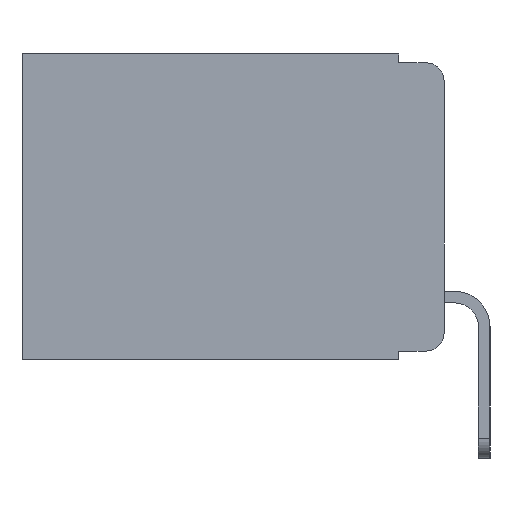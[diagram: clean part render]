
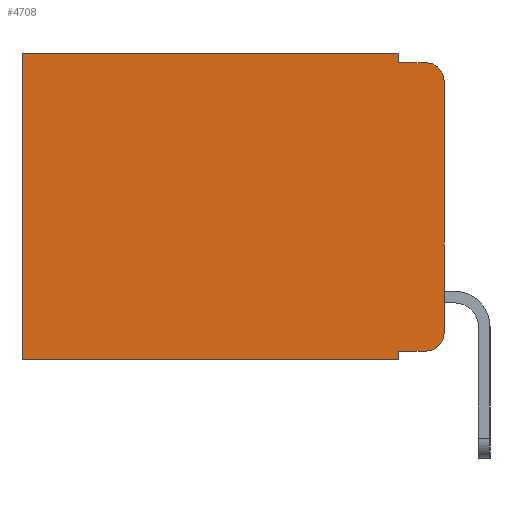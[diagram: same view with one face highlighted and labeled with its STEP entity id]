
A CAD part, left-side view. The second image highlights one B-rep face of the part: STEP entity #4708.
In plain terms, the highlighted planar face has unit normal (-1, 0, 0).
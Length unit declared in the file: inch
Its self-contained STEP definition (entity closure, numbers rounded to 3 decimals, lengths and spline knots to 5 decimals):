
#97 = VERTEX_POINT ( 'NONE', #3400 ) ;
#129 = EDGE_CURVE ( 'NONE', #6507, #97, #11441, .T. ) ;
#184 = VECTOR ( 'NONE', #4500, 39.37008 ) ;
#549 = CARTESIAN_POINT ( 'NONE',  ( 0.298, 0.02, -0.03 ) ) ;
#659 = CARTESIAN_POINT ( 'NONE',  ( 0.298, 0.473, 0. ) ) ;
#686 = LINE ( 'NONE', #10737, #2802 ) ;
#793 = CARTESIAN_POINT ( 'NONE',  ( 0.298, 0.051, -0.333 ) ) ;
#850 = EDGE_CURVE ( 'NONE', #11852, #7613, #6948, .T. ) ;
#1133 = VERTEX_POINT ( 'NONE', #4313 ) ;
#1207 = CARTESIAN_POINT ( 'NONE',  ( 0.298, 0.051, -0.01 ) ) ;
#1208 = VECTOR ( 'NONE', #5423, 39.37008 ) ;
#1633 = ORIENTED_EDGE ( 'NONE', *, *, #5305, .F. ) ;
#1753 = EDGE_CURVE ( 'NONE', #10058, #8512, #686, .T. ) ;
#1862 = LINE ( 'NONE', #9251, #4574 ) ;
#1999 = DIRECTION ( 'NONE',  ( 0., 0., -1. ) ) ;
#2499 = DIRECTION ( 'NONE',  ( 0., 0., -1. ) ) ;
#2802 = VECTOR ( 'NONE', #3486, 39.37008 ) ;
#3192 = CARTESIAN_POINT ( 'NONE',  ( 0.298, 0.02, -0.333 ) ) ;
#3314 = LINE ( 'NONE', #1207, #184 ) ;
#3400 = CARTESIAN_POINT ( 'NONE',  ( 0.298, 0.02, -0.01 ) ) ;
#3486 = DIRECTION ( 'NONE',  ( 0., 1., 0. ) ) ;
#3819 = FACE_OUTER_BOUND ( 'NONE', #6431, .T. ) ;
#3943 = LINE ( 'NONE', #5377, #1208 ) ;
#3947 = LINE ( 'NONE', #11759, #9276 ) ;
#4313 = CARTESIAN_POINT ( 'NONE',  ( 0.298, 0.051, 0. ) ) ;
#4397 = CARTESIAN_POINT ( 'NONE',  ( 0.298, 0.473, 0. ) ) ;
#4480 = LINE ( 'NONE', #5407, #11671 ) ;
#4500 = DIRECTION ( 'NONE',  ( 0., -1., 0. ) ) ;
#4574 = VECTOR ( 'NONE', #4771, 39.37008 ) ;
#4708 = ADVANCED_FACE ( 'NONE', ( #3819 ), #8850, .F. ) ;
#4771 = DIRECTION ( 'NONE',  ( 0., 0., -1. ) ) ;
#4872 = CARTESIAN_POINT ( 'NONE',  ( 0.298, 0., -0.03 ) ) ;
#4973 = EDGE_CURVE ( 'NONE', #10685, #8512, #10595, .T. ) ;
#5069 = EDGE_CURVE ( 'NONE', #1133, #10685, #3947, .T. ) ;
#5122 = EDGE_CURVE ( 'NONE', #11947, #97, #3314, .T. ) ;
#5305 = EDGE_CURVE ( 'NONE', #8249, #10058, #1862, .T. ) ;
#5351 = CARTESIAN_POINT ( 'NONE',  ( 0.298, 0.051, -0.01 ) ) ;
#5377 = CARTESIAN_POINT ( 'NONE',  ( 0.298, 0.051, -0.333 ) ) ;
#5407 = CARTESIAN_POINT ( 'NONE',  ( 0.298, 0., 0. ) ) ;
#5423 = DIRECTION ( 'NONE',  ( 0., -1., 0. ) ) ;
#5557 = EDGE_CURVE ( 'NONE', #6507, #7613, #4480, .T. ) ;
#6135 = CARTESIAN_POINT ( 'NONE',  ( 0.298, 0.473, -0.343 ) ) ;
#6237 = CARTESIAN_POINT ( 'NONE',  ( 0.298, 0.051, -0.343 ) ) ;
#6258 = AXIS2_PLACEMENT_3D ( 'NONE', #8302, #11763, #2499 ) ;
#6431 = EDGE_LOOP ( 'NONE', ( #8697, #10880, #6558, #11122, #9213, #9472, #6723, #1633, #7314, #9881 ) ) ;
#6507 = VERTEX_POINT ( 'NONE', #4872 ) ;
#6558 = ORIENTED_EDGE ( 'NONE', *, *, #5122, .F. ) ;
#6723 = ORIENTED_EDGE ( 'NONE', *, *, #1753, .F. ) ;
#6948 = CIRCLE ( 'NONE', #6258, 0.02 ) ;
#7032 = CARTESIAN_POINT ( 'NONE',  ( 0.298, 0.051, 0. ) ) ;
#7193 = DIRECTION ( 'NONE',  ( 0., 0., -1. ) ) ;
#7314 = ORIENTED_EDGE ( 'NONE', *, *, #10292, .T. ) ;
#7613 = VERTEX_POINT ( 'NONE', #10015 ) ;
#8249 = VERTEX_POINT ( 'NONE', #793 ) ;
#8302 = CARTESIAN_POINT ( 'NONE',  ( 0.298, 0.02, -0.313 ) ) ;
#8512 = VERTEX_POINT ( 'NONE', #6135 ) ;
#8697 = ORIENTED_EDGE ( 'NONE', *, *, #5557, .F. ) ;
#8727 = AXIS2_PLACEMENT_3D ( 'NONE', #8780, #9002, #8937 ) ;
#8780 = CARTESIAN_POINT ( 'NONE',  ( 0.298, 0., 0. ) ) ;
#8850 = PLANE ( 'NONE',  #8727 ) ;
#8910 = AXIS2_PLACEMENT_3D ( 'NONE', #549, #9350, #9328 ) ;
#8937 = DIRECTION ( 'NONE',  ( 0., 0., -1. ) ) ;
#9002 = DIRECTION ( 'NONE',  ( 1., 0., 0. ) ) ;
#9213 = ORIENTED_EDGE ( 'NONE', *, *, #5069, .T. ) ;
#9251 = CARTESIAN_POINT ( 'NONE',  ( 0.298, 0.051, 0. ) ) ;
#9276 = VECTOR ( 'NONE', #11627, 39.37008 ) ;
#9328 = DIRECTION ( 'NONE',  ( 0., 0., -1. ) ) ;
#9350 = DIRECTION ( 'NONE',  ( -1., 0., 0. ) ) ;
#9472 = ORIENTED_EDGE ( 'NONE', *, *, #4973, .T. ) ;
#9881 = ORIENTED_EDGE ( 'NONE', *, *, #850, .T. ) ;
#10015 = CARTESIAN_POINT ( 'NONE',  ( 0.298, 0., -0.313 ) ) ;
#10058 = VERTEX_POINT ( 'NONE', #6237 ) ;
#10292 = EDGE_CURVE ( 'NONE', #8249, #11852, #3943, .T. ) ;
#10595 = LINE ( 'NONE', #4397, #10833 ) ;
#10685 = VERTEX_POINT ( 'NONE', #659 ) ;
#10694 = VECTOR ( 'NONE', #1999, 39.37008 ) ;
#10737 = CARTESIAN_POINT ( 'NONE',  ( 0.298, 0., -0.343 ) ) ;
#10775 = DIRECTION ( 'NONE',  ( 0., 0., -1. ) ) ;
#10833 = VECTOR ( 'NONE', #7193, 39.37008 ) ;
#10880 = ORIENTED_EDGE ( 'NONE', *, *, #129, .T. ) ;
#10931 = LINE ( 'NONE', #7032, #10694 ) ;
#10939 = EDGE_CURVE ( 'NONE', #1133, #11947, #10931, .T. ) ;
#11122 = ORIENTED_EDGE ( 'NONE', *, *, #10939, .F. ) ;
#11441 = CIRCLE ( 'NONE', #8910, 0.02 ) ;
#11627 = DIRECTION ( 'NONE',  ( 0., 1., 0. ) ) ;
#11671 = VECTOR ( 'NONE', #10775, 39.37008 ) ;
#11759 = CARTESIAN_POINT ( 'NONE',  ( 0.298, 0., 0. ) ) ;
#11763 = DIRECTION ( 'NONE',  ( -1., 0., 0. ) ) ;
#11852 = VERTEX_POINT ( 'NONE', #3192 ) ;
#11947 = VERTEX_POINT ( 'NONE', #5351 ) ;
